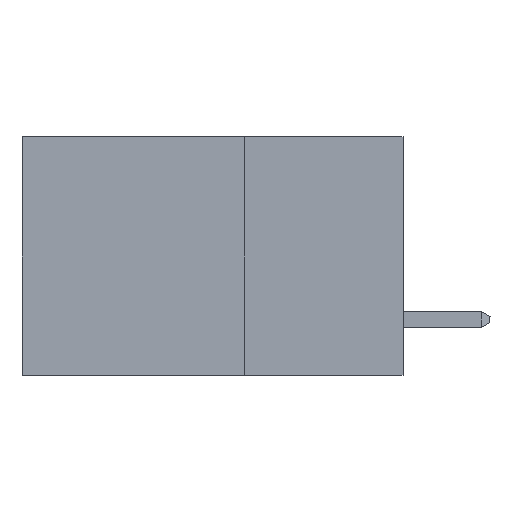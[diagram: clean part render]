
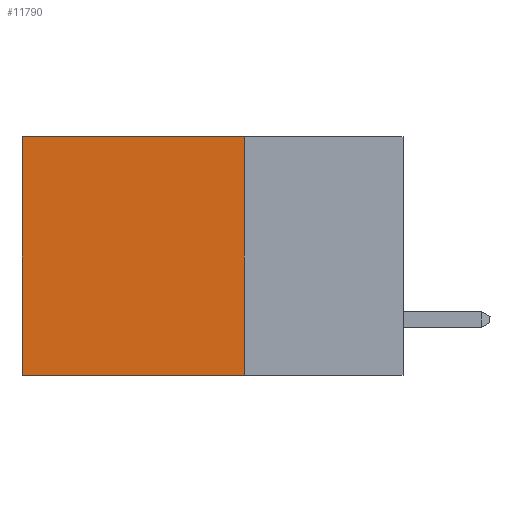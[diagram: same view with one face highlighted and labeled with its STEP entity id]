
A CAD part, left-side view. The second image highlights one B-rep face of the part: STEP entity #11790.
In plain terms, the highlighted planar face has unit normal (-1, 0, 0).
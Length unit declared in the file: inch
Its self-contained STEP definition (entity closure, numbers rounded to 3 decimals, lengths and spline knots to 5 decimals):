
#208 = DIRECTION ( 'NONE',  ( 0., 1., 0. ) ) ;
#808 = EDGE_CURVE ( 'NONE', #4306, #12620, #12202, .T. ) ;
#1272 = CARTESIAN_POINT ( 'NONE',  ( 0.2875, 0.25, -0.375 ) ) ;
#2445 = LINE ( 'NONE', #12483, #6664 ) ;
#2449 = CARTESIAN_POINT ( 'NONE',  ( 0.2875, 0.25, -0.375 ) ) ;
#2455 = DIRECTION ( 'NONE',  ( 0., 0., -1. ) ) ;
#2915 = PLANE ( 'NONE',  #8383 ) ;
#3528 = VECTOR ( 'NONE', #3554, 39.37008 ) ;
#3554 = DIRECTION ( 'NONE',  ( 0., 1., 0. ) ) ;
#3933 = DIRECTION ( 'NONE',  ( 1., 0., 0. ) ) ;
#4306 = VERTEX_POINT ( 'NONE', #14037 ) ;
#4793 = LINE ( 'NONE', #13521, #3528 ) ;
#5462 = ORIENTED_EDGE ( 'NONE', *, *, #5929, .F. ) ;
#5738 = CARTESIAN_POINT ( 'NONE',  ( 0.2875, 0.6, -0.375 ) ) ;
#5852 = LINE ( 'NONE', #1272, #7034 ) ;
#5929 = EDGE_CURVE ( 'NONE', #10137, #12620, #4793, .T. ) ;
#6054 = FACE_OUTER_BOUND ( 'NONE', #12759, .T. ) ;
#6076 = CARTESIAN_POINT ( 'NONE',  ( 0.2875, 0.6, -0.375 ) ) ;
#6268 = CARTESIAN_POINT ( 'NONE',  ( 0.2875, 0.25, -0.375 ) ) ;
#6664 = VECTOR ( 'NONE', #208, 39.37008 ) ;
#6943 = DIRECTION ( 'NONE',  ( 0., 0., -1. ) ) ;
#7034 = VECTOR ( 'NONE', #6943, 39.37008 ) ;
#7539 = EDGE_CURVE ( 'NONE', #13835, #10137, #5852, .T. ) ;
#8383 = AXIS2_PLACEMENT_3D ( 'NONE', #6268, #3933, #9616 ) ;
#8464 = EDGE_CURVE ( 'NONE', #13835, #4306, #2445, .T. ) ;
#9126 = VECTOR ( 'NONE', #2455, 39.37008 ) ;
#9494 = ORIENTED_EDGE ( 'NONE', *, *, #7539, .F. ) ;
#9616 = DIRECTION ( 'NONE',  ( 0., 0., -1. ) ) ;
#10137 = VERTEX_POINT ( 'NONE', #2449 ) ;
#11790 = ADVANCED_FACE ( 'NONE', ( #6054 ), #2915, .F. ) ;
#12154 = ORIENTED_EDGE ( 'NONE', *, *, #808, .T. ) ;
#12202 = LINE ( 'NONE', #5738, #9126 ) ;
#12483 = CARTESIAN_POINT ( 'NONE',  ( 0.2875, 0.25, 0. ) ) ;
#12620 = VERTEX_POINT ( 'NONE', #6076 ) ;
#12759 = EDGE_LOOP ( 'NONE', ( #12154, #5462, #9494, #12774 ) ) ;
#12774 = ORIENTED_EDGE ( 'NONE', *, *, #8464, .T. ) ;
#13295 = CARTESIAN_POINT ( 'NONE',  ( 0.2875, 0.25, 0. ) ) ;
#13521 = CARTESIAN_POINT ( 'NONE',  ( 0.2875, 0.25, -0.375 ) ) ;
#13835 = VERTEX_POINT ( 'NONE', #13295 ) ;
#14037 = CARTESIAN_POINT ( 'NONE',  ( 0.2875, 0.6, 0. ) ) ;
